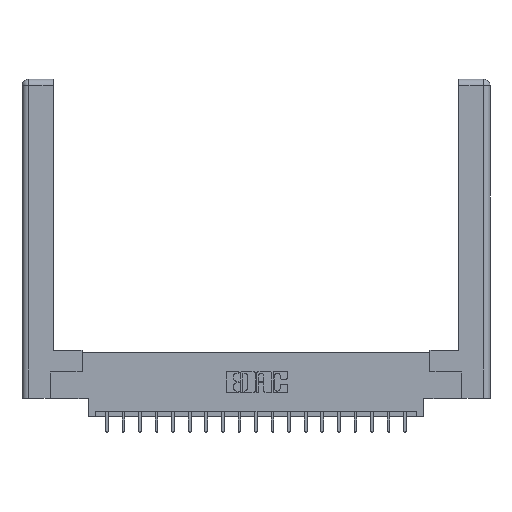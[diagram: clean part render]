
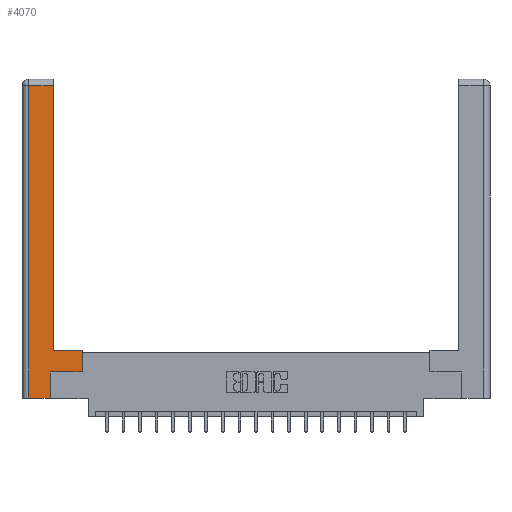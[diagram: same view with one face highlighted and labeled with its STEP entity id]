
A CAD part, top view. The second image highlights one B-rep face of the part: STEP entity #4070.
In plain terms, the highlighted planar face has unit normal (0, 0, 1).
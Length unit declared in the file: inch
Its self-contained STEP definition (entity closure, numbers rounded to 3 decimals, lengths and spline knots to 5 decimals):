
#399 = DIRECTION ( 'NONE',  ( 0., 1., 0. ) ) ;
#760 = DIRECTION ( 'NONE',  ( 0., 1., 0. ) ) ;
#943 = VECTOR ( 'NONE', #760, 39.37008 ) ;
#1286 = EDGE_CURVE ( 'NONE', #10831, #3229, #1478, .T. ) ;
#1478 = LINE ( 'NONE', #6753, #5730 ) ;
#1554 = CARTESIAN_POINT ( 'NONE',  ( 0.265, 0., 0. ) ) ;
#1998 = VECTOR ( 'NONE', #17427, 39.37008 ) ;
#2163 = DIRECTION ( 'NONE',  ( 1., 0., 0. ) ) ;
#2442 = LINE ( 'NONE', #2567, #943 ) ;
#2567 = CARTESIAN_POINT ( 'NONE',  ( 0.265, 0.245, 0. ) ) ;
#2694 = CARTESIAN_POINT ( 'NONE',  ( 0.295, 2.94, 0. ) ) ;
#3229 = VERTEX_POINT ( 'NONE', #10468 ) ;
#3385 = CARTESIAN_POINT ( 'NONE',  ( 0.0615, 2.94, 0. ) ) ;
#3449 = CARTESIAN_POINT ( 'NONE',  ( 0.0615, 0., 0. ) ) ;
#4070 = ADVANCED_FACE ( 'NONE', ( #13491 ), #9454, .F. ) ;
#4933 = EDGE_CURVE ( 'NONE', #19767, #13732, #9098, .T. ) ;
#5047 = DIRECTION ( 'NONE',  ( -1., 0., 0. ) ) ;
#5494 = VECTOR ( 'NONE', #2163, 39.37008 ) ;
#5730 = VECTOR ( 'NONE', #399, 39.37008 ) ;
#5812 = VECTOR ( 'NONE', #17242, 39.37008 ) ;
#5943 = VECTOR ( 'NONE', #16636, 39.37008 ) ;
#6230 = CARTESIAN_POINT ( 'NONE',  ( 0.265, 0., 0. ) ) ;
#6481 = CARTESIAN_POINT ( 'NONE',  ( 0.295, 3., 0. ) ) ;
#6753 = CARTESIAN_POINT ( 'NONE',  ( 0.565, 0.45, 0. ) ) ;
#7045 = CARTESIAN_POINT ( 'NONE',  ( 0.565, 0.245, 0. ) ) ;
#7341 = ORIENTED_EDGE ( 'NONE', *, *, #4933, .T. ) ;
#7874 = ORIENTED_EDGE ( 'NONE', *, *, #17657, .T. ) ;
#7969 = LINE ( 'NONE', #16621, #17593 ) ;
#8081 = CARTESIAN_POINT ( 'NONE',  ( 0., 0., 0. ) ) ;
#8728 = DIRECTION ( 'NONE',  ( -1., 0., 0. ) ) ;
#9068 = ORIENTED_EDGE ( 'NONE', *, *, #14311, .T. ) ;
#9098 = LINE ( 'NONE', #10481, #9599 ) ;
#9347 = ORIENTED_EDGE ( 'NONE', *, *, #15450, .T. ) ;
#9454 = PLANE ( 'NONE',  #13076 ) ;
#9486 = LINE ( 'NONE', #6230, #5812 ) ;
#9599 = VECTOR ( 'NONE', #15192, 39.37008 ) ;
#10334 = VERTEX_POINT ( 'NONE', #19620 ) ;
#10424 = VERTEX_POINT ( 'NONE', #2694 ) ;
#10468 = CARTESIAN_POINT ( 'NONE',  ( 0.565, 0.45, 0. ) ) ;
#10481 = CARTESIAN_POINT ( 'NONE',  ( 0.0615, 0., 0. ) ) ;
#10831 = VERTEX_POINT ( 'NONE', #7045 ) ;
#11048 = LINE ( 'NONE', #11886, #5943 ) ;
#11084 = ORIENTED_EDGE ( 'NONE', *, *, #1286, .T. ) ;
#11466 = EDGE_CURVE ( 'NONE', #10424, #19767, #7969, .T. ) ;
#11656 = CARTESIAN_POINT ( 'NONE',  ( 0.565, 0.245, 0. ) ) ;
#11779 = VERTEX_POINT ( 'NONE', #1554 ) ;
#11886 = CARTESIAN_POINT ( 'NONE',  ( 0.295, 0.45, 0. ) ) ;
#12254 = EDGE_LOOP ( 'NONE', ( #9068, #15532, #7341, #17310, #7874, #9347, #11084, #17203 ) ) ;
#12589 = LINE ( 'NONE', #6481, #1998 ) ;
#13076 = AXIS2_PLACEMENT_3D ( 'NONE', #8081, #14553, #5047 ) ;
#13491 = FACE_OUTER_BOUND ( 'NONE', #12254, .T. ) ;
#13732 = VERTEX_POINT ( 'NONE', #3449 ) ;
#13937 = EDGE_CURVE ( 'NONE', #3229, #19243, #11048, .T. ) ;
#14311 = EDGE_CURVE ( 'NONE', #19243, #10424, #12589, .T. ) ;
#14553 = DIRECTION ( 'NONE',  ( 0., 0., -1. ) ) ;
#14698 = CARTESIAN_POINT ( 'NONE',  ( 0.295, 0.45, 0. ) ) ;
#15192 = DIRECTION ( 'NONE',  ( 0., -1., 0. ) ) ;
#15450 = EDGE_CURVE ( 'NONE', #10334, #10831, #18313, .T. ) ;
#15532 = ORIENTED_EDGE ( 'NONE', *, *, #11466, .T. ) ;
#16621 = CARTESIAN_POINT ( 'NONE',  ( 0.0615, 2.94, 0. ) ) ;
#16636 = DIRECTION ( 'NONE',  ( -1., 0., 0. ) ) ;
#17203 = ORIENTED_EDGE ( 'NONE', *, *, #13937, .T. ) ;
#17242 = DIRECTION ( 'NONE',  ( 1., 0., 0. ) ) ;
#17310 = ORIENTED_EDGE ( 'NONE', *, *, #20178, .T. ) ;
#17427 = DIRECTION ( 'NONE',  ( 0., 1., 0. ) ) ;
#17593 = VECTOR ( 'NONE', #8728, 39.37008 ) ;
#17657 = EDGE_CURVE ( 'NONE', #11779, #10334, #2442, .T. ) ;
#18313 = LINE ( 'NONE', #11656, #5494 ) ;
#19243 = VERTEX_POINT ( 'NONE', #14698 ) ;
#19620 = CARTESIAN_POINT ( 'NONE',  ( 0.265, 0.245, 0. ) ) ;
#19767 = VERTEX_POINT ( 'NONE', #3385 ) ;
#20178 = EDGE_CURVE ( 'NONE', #13732, #11779, #9486, .T. ) ;
